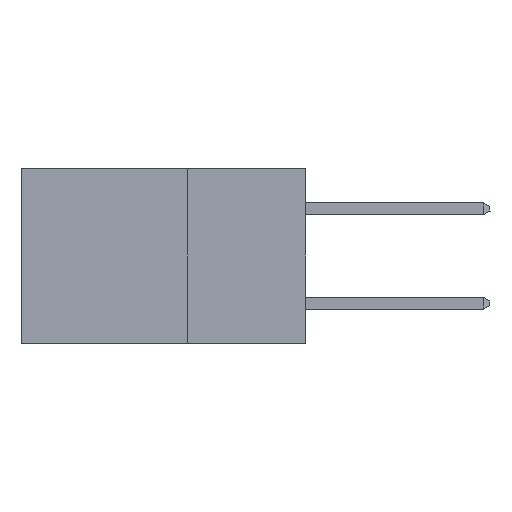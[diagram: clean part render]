
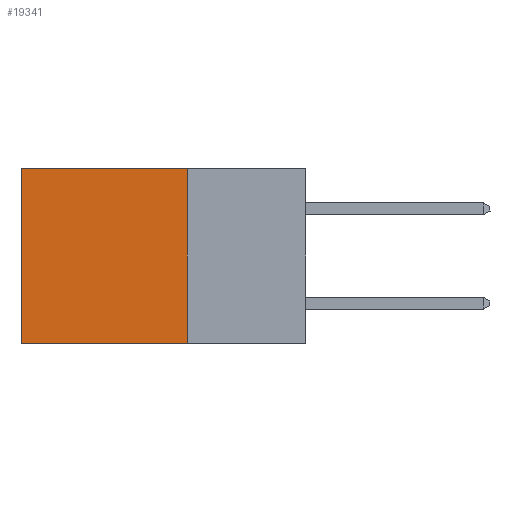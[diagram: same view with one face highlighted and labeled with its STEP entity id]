
A CAD part, left-side view. The second image highlights one B-rep face of the part: STEP entity #19341.
In plain terms, the highlighted planar face has unit normal (-1, 0, 0).
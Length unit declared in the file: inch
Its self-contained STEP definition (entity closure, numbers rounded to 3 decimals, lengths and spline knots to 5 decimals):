
#1142 = LINE ( 'NONE', #16853, #10283 ) ;
#1178 = CARTESIAN_POINT ( 'NONE',  ( 0.298, 0.25, 0. ) ) ;
#6025 = DIRECTION ( 'NONE',  ( 0., 1., 0. ) ) ;
#6822 = EDGE_CURVE ( 'NONE', #9597, #16898, #8632, .T. ) ;
#7744 = EDGE_CURVE ( 'NONE', #19127, #12899, #1142, .T. ) ;
#8613 = ORIENTED_EDGE ( 'NONE', *, *, #7744, .T. ) ;
#8632 = LINE ( 'NONE', #27004, #14188 ) ;
#8910 = CARTESIAN_POINT ( 'NONE',  ( 0.298, 0.6, 0. ) ) ;
#9366 = DIRECTION ( 'NONE',  ( 0., 0., -1. ) ) ;
#9597 = VERTEX_POINT ( 'NONE', #20538 ) ;
#9899 = AXIS2_PLACEMENT_3D ( 'NONE', #1178, #15253, #19999 ) ;
#10283 = VECTOR ( 'NONE', #16646, 39.37008 ) ;
#11405 = ORIENTED_EDGE ( 'NONE', *, *, #25885, .T. ) ;
#11496 = DIRECTION ( 'NONE',  ( 0., 0., -1. ) ) ;
#11758 = ORIENTED_EDGE ( 'NONE', *, *, #6822, .F. ) ;
#12899 = VERTEX_POINT ( 'NONE', #14663 ) ;
#13924 = EDGE_CURVE ( 'NONE', #19127, #9597, #19452, .T. ) ;
#13932 = VECTOR ( 'NONE', #9366, 39.37008 ) ;
#14188 = VECTOR ( 'NONE', #6025, 39.37008 ) ;
#14663 = CARTESIAN_POINT ( 'NONE',  ( 0.298, 0.6, 0. ) ) ;
#15253 = DIRECTION ( 'NONE',  ( 1., 0., 0. ) ) ;
#16138 = EDGE_LOOP ( 'NONE', ( #11405, #11758, #21396, #8613 ) ) ;
#16646 = DIRECTION ( 'NONE',  ( 0., 1., 0. ) ) ;
#16853 = CARTESIAN_POINT ( 'NONE',  ( 0.298, 0.25, 0. ) ) ;
#16898 = VERTEX_POINT ( 'NONE', #20992 ) ;
#17722 = PLANE ( 'NONE',  #9899 ) ;
#19127 = VERTEX_POINT ( 'NONE', #20205 ) ;
#19341 = ADVANCED_FACE ( 'NONE', ( #26538 ), #17722, .F. ) ;
#19452 = LINE ( 'NONE', #21044, #13932 ) ;
#19999 = DIRECTION ( 'NONE',  ( 0., 0., -1. ) ) ;
#20205 = CARTESIAN_POINT ( 'NONE',  ( 0.298, 0.25, 0. ) ) ;
#20538 = CARTESIAN_POINT ( 'NONE',  ( 0.298, 0.25, -0.37 ) ) ;
#20992 = CARTESIAN_POINT ( 'NONE',  ( 0.298, 0.6, -0.37 ) ) ;
#21044 = CARTESIAN_POINT ( 'NONE',  ( 0.298, 0.25, 0. ) ) ;
#21396 = ORIENTED_EDGE ( 'NONE', *, *, #13924, .F. ) ;
#23543 = VECTOR ( 'NONE', #11496, 39.37008 ) ;
#25885 = EDGE_CURVE ( 'NONE', #12899, #16898, #30543, .T. ) ;
#26538 = FACE_OUTER_BOUND ( 'NONE', #16138, .T. ) ;
#27004 = CARTESIAN_POINT ( 'NONE',  ( 0.298, 0.25, -0.37 ) ) ;
#30543 = LINE ( 'NONE', #8910, #23543 ) ;
